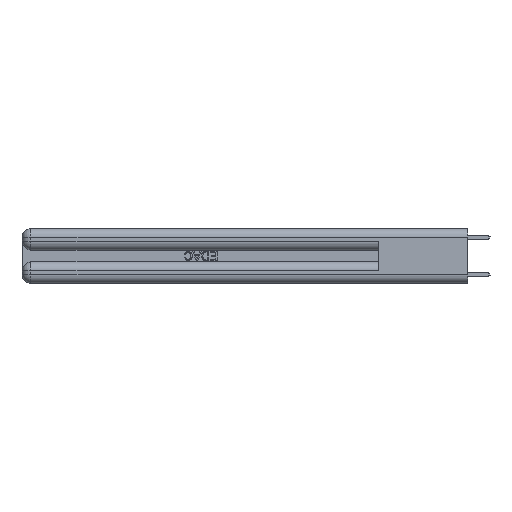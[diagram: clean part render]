
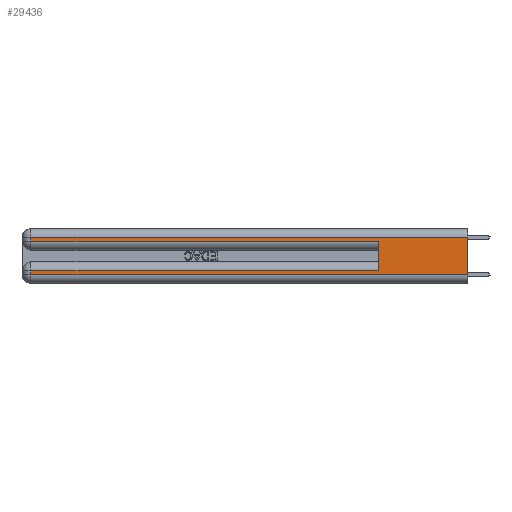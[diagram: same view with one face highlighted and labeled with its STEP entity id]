
A CAD part, left-side view. The second image highlights one B-rep face of the part: STEP entity #29436.
In plain terms, the highlighted planar face has unit normal (-1, 0, 0).
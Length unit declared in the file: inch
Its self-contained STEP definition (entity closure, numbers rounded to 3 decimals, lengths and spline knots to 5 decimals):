
#1277 = EDGE_CURVE ( 'NONE', #12546, #21331, #9539, .T. ) ;
#1509 = EDGE_LOOP ( 'NONE', ( #4822, #2509, #9837, #14446, #14309, #14834, #24158, #7053 ) ) ;
#1799 = LINE ( 'NONE', #33172, #16374 ) ;
#1870 = LINE ( 'NONE', #35847, #18636 ) ;
#2019 = DIRECTION ( 'NONE',  ( 0., 0., -1. ) ) ;
#2509 = ORIENTED_EDGE ( 'NONE', *, *, #15855, .T. ) ;
#3047 = LINE ( 'NONE', #31452, #5464 ) ;
#4822 = ORIENTED_EDGE ( 'NONE', *, *, #17028, .F. ) ;
#5464 = VECTOR ( 'NONE', #31281, 39.37008 ) ;
#5561 = LINE ( 'NONE', #13921, #16892 ) ;
#6408 = VERTEX_POINT ( 'NONE', #22798 ) ;
#6937 = DIRECTION ( 'NONE',  ( 0., 0., 1. ) ) ;
#7053 = ORIENTED_EDGE ( 'NONE', *, *, #28227, .T. ) ;
#8246 = LINE ( 'NONE', #19556, #10003 ) ;
#8348 = CARTESIAN_POINT ( 'NONE',  ( 0., 0., 0.37 ) ) ;
#8723 = CARTESIAN_POINT ( 'NONE',  ( 0., 2.94, 0.37 ) ) ;
#8754 = LINE ( 'NONE', #11541, #23919 ) ;
#9539 = LINE ( 'NONE', #32361, #32680 ) ;
#9569 = CARTESIAN_POINT ( 'NONE',  ( 0., 2.94, 0.285 ) ) ;
#9837 = ORIENTED_EDGE ( 'NONE', *, *, #33389, .T. ) ;
#9956 = CARTESIAN_POINT ( 'NONE',  ( 0., 0.6, 0.285 ) ) ;
#10003 = VECTOR ( 'NONE', #19937, 39.37008 ) ;
#10243 = EDGE_CURVE ( 'NONE', #35120, #18620, #11509, .T. ) ;
#10432 = DIRECTION ( 'NONE',  ( 0., 0., -1. ) ) ;
#11509 = LINE ( 'NONE', #8723, #27276 ) ;
#11510 = DIRECTION ( 'NONE',  ( 0., 0., -1. ) ) ;
#11541 = CARTESIAN_POINT ( 'NONE',  ( 0., 0., 0.31 ) ) ;
#12546 = VERTEX_POINT ( 'NONE', #18322 ) ;
#12937 = VERTEX_POINT ( 'NONE', #29061 ) ;
#13921 = CARTESIAN_POINT ( 'NONE',  ( 0., 2.94, 0.37 ) ) ;
#14309 = ORIENTED_EDGE ( 'NONE', *, *, #1277, .F. ) ;
#14446 = ORIENTED_EDGE ( 'NONE', *, *, #34985, .T. ) ;
#14834 = ORIENTED_EDGE ( 'NONE', *, *, #36274, .T. ) ;
#15855 = EDGE_CURVE ( 'NONE', #30005, #12937, #8754, .T. ) ;
#16374 = VECTOR ( 'NONE', #18346, 39.37008 ) ;
#16892 = VECTOR ( 'NONE', #11510, 39.37008 ) ;
#17028 = EDGE_CURVE ( 'NONE', #30005, #6408, #1870, .T. ) ;
#18322 = CARTESIAN_POINT ( 'NONE',  ( 0., 0.6, 0.085 ) ) ;
#18346 = DIRECTION ( 'NONE',  ( 0., -1., 0. ) ) ;
#18620 = VERTEX_POINT ( 'NONE', #29524 ) ;
#18636 = VECTOR ( 'NONE', #10432, 39.37008 ) ;
#19556 = CARTESIAN_POINT ( 'NONE',  ( 0., 0., 0.085 ) ) ;
#19937 = DIRECTION ( 'NONE',  ( 0., 1., 0. ) ) ;
#21331 = VERTEX_POINT ( 'NONE', #9956 ) ;
#22461 = PLANE ( 'NONE',  #26878 ) ;
#22798 = CARTESIAN_POINT ( 'NONE',  ( 0., 0., 0.06 ) ) ;
#23041 = DIRECTION ( 'NONE',  ( 0., 1., 0. ) ) ;
#23919 = VECTOR ( 'NONE', #23041, 39.37008 ) ;
#24158 = ORIENTED_EDGE ( 'NONE', *, *, #10243, .T. ) ;
#26347 = DIRECTION ( 'NONE',  ( 0., 0., -1. ) ) ;
#26557 = VERTEX_POINT ( 'NONE', #9569 ) ;
#26878 = AXIS2_PLACEMENT_3D ( 'NONE', #8348, #27830, #2019 ) ;
#26959 = CARTESIAN_POINT ( 'NONE',  ( 0., 2.94, 0.085 ) ) ;
#27276 = VECTOR ( 'NONE', #26347, 39.37008 ) ;
#27830 = DIRECTION ( 'NONE',  ( 1., 0., 0. ) ) ;
#28227 = EDGE_CURVE ( 'NONE', #18620, #6408, #3047, .T. ) ;
#29061 = CARTESIAN_POINT ( 'NONE',  ( 0., 2.94, 0.31 ) ) ;
#29436 = ADVANCED_FACE ( 'NONE', ( #33026 ), #22461, .F. ) ;
#29524 = CARTESIAN_POINT ( 'NONE',  ( 0., 2.94, 0.06 ) ) ;
#30005 = VERTEX_POINT ( 'NONE', #31317 ) ;
#31281 = DIRECTION ( 'NONE',  ( 0., -1., 0. ) ) ;
#31317 = CARTESIAN_POINT ( 'NONE',  ( 0., 0., 0.31 ) ) ;
#31452 = CARTESIAN_POINT ( 'NONE',  ( 0., 0., 0.06 ) ) ;
#32361 = CARTESIAN_POINT ( 'NONE',  ( 0., 0.6, 0.145 ) ) ;
#32680 = VECTOR ( 'NONE', #6937, 39.37008 ) ;
#33026 = FACE_OUTER_BOUND ( 'NONE', #1509, .T. ) ;
#33172 = CARTESIAN_POINT ( 'NONE',  ( 0., 0., 0.285 ) ) ;
#33389 = EDGE_CURVE ( 'NONE', #12937, #26557, #5561, .T. ) ;
#34985 = EDGE_CURVE ( 'NONE', #26557, #21331, #1799, .T. ) ;
#35120 = VERTEX_POINT ( 'NONE', #26959 ) ;
#35847 = CARTESIAN_POINT ( 'NONE',  ( 0., 0., 0.37 ) ) ;
#36274 = EDGE_CURVE ( 'NONE', #12546, #35120, #8246, .T. ) ;
